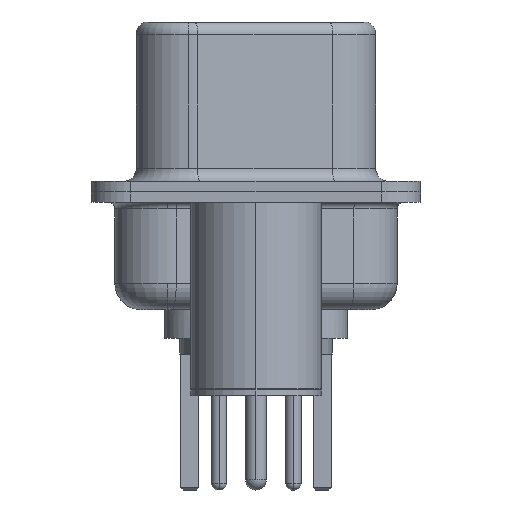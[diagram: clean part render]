
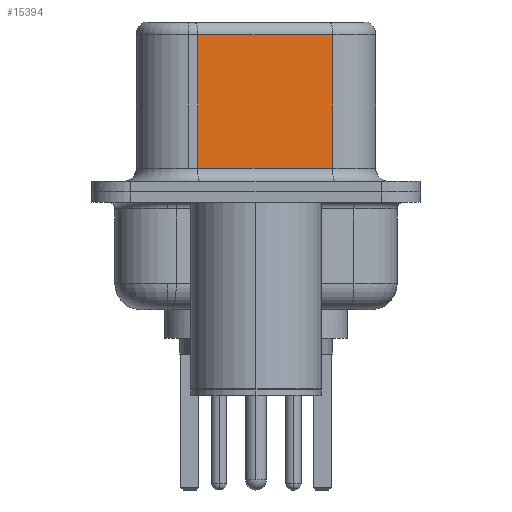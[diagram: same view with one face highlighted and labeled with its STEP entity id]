
A CAD part, left-side view. The second image highlights one B-rep face of the part: STEP entity #15394.
In plain terms, the highlighted planar face has unit normal (-0.985, -0.174, 0).
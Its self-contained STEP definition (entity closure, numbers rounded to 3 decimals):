
#311 = DIRECTION ( 'NONE',  ( 0., 0., -1. ) ) ;
#354 = VECTOR ( 'NONE', #311, 1000. ) ;
#778 = VECTOR ( 'NONE', #16590, 1000. ) ;
#816 = EDGE_CURVE ( 'NONE', #8289, #9827, #10720, .T. ) ;
#1275 = ORIENTED_EDGE ( 'NONE', *, *, #15226, .T. ) ;
#1513 = DIRECTION ( 'NONE',  ( -0.174, 0.985, 0. ) ) ;
#2016 = LINE ( 'NONE', #14403, #16893 ) ;
#4071 = LINE ( 'NONE', #24853, #8042 ) ;
#5916 = CARTESIAN_POINT ( 'NONE',  ( 4.585, -2.927, 6.52 ) ) ;
#6056 = VERTEX_POINT ( 'NONE', #23056 ) ;
#6843 = ORIENTED_EDGE ( 'NONE', *, *, #23059, .T. ) ;
#6895 = CARTESIAN_POINT ( 'NONE',  ( 3.675, 2.233, 6.52 ) ) ;
#7898 = PLANE ( 'NONE',  #8907 ) ;
#8042 = VECTOR ( 'NONE', #1513, 1000. ) ;
#8288 = ORIENTED_EDGE ( 'NONE', *, *, #816, .T. ) ;
#8289 = VERTEX_POINT ( 'NONE', #21233 ) ;
#8363 = EDGE_LOOP ( 'NONE', ( #24062, #1275, #8288, #6843 ) ) ;
#8907 = AXIS2_PLACEMENT_3D ( 'NONE', #5916, #21402, #9856 ) ;
#9827 = VERTEX_POINT ( 'NONE', #16968 ) ;
#9856 = DIRECTION ( 'NONE',  ( -0.174, 0.985, 0. ) ) ;
#10720 = LINE ( 'NONE', #6895, #354 ) ;
#13762 = VERTEX_POINT ( 'NONE', #24611 ) ;
#14403 = CARTESIAN_POINT ( 'NONE',  ( 4.585, -2.927, 0.9 ) ) ;
#15226 = EDGE_CURVE ( 'NONE', #6056, #8289, #4071, .T. ) ;
#15394 = ADVANCED_FACE ( 'NONE', ( #20420 ), #7898, .F. ) ;
#16590 = DIRECTION ( 'NONE',  ( 0., 0., -1. ) ) ;
#16863 = LINE ( 'NONE', #20447, #778 ) ;
#16893 = VECTOR ( 'NONE', #18200, 1000. ) ;
#16968 = CARTESIAN_POINT ( 'NONE',  ( 3.675, 2.233, 0.9 ) ) ;
#18200 = DIRECTION ( 'NONE',  ( 0.174, -0.985, 0. ) ) ;
#20420 = FACE_OUTER_BOUND ( 'NONE', #8363, .T. ) ;
#20447 = CARTESIAN_POINT ( 'NONE',  ( 4.585, -2.927, 6.52 ) ) ;
#21233 = CARTESIAN_POINT ( 'NONE',  ( 3.675, 2.233, 6.02 ) ) ;
#21402 = DIRECTION ( 'NONE',  ( 0.985, 0.174, 0. ) ) ;
#23056 = CARTESIAN_POINT ( 'NONE',  ( 4.585, -2.927, 6.02 ) ) ;
#23059 = EDGE_CURVE ( 'NONE', #9827, #13762, #2016, .T. ) ;
#23699 = EDGE_CURVE ( 'NONE', #6056, #13762, #16863, .T. ) ;
#24062 = ORIENTED_EDGE ( 'NONE', *, *, #23699, .F. ) ;
#24611 = CARTESIAN_POINT ( 'NONE',  ( 4.585, -2.927, 0.9 ) ) ;
#24853 = CARTESIAN_POINT ( 'NONE',  ( 4.585, -2.927, 6.02 ) ) ;
